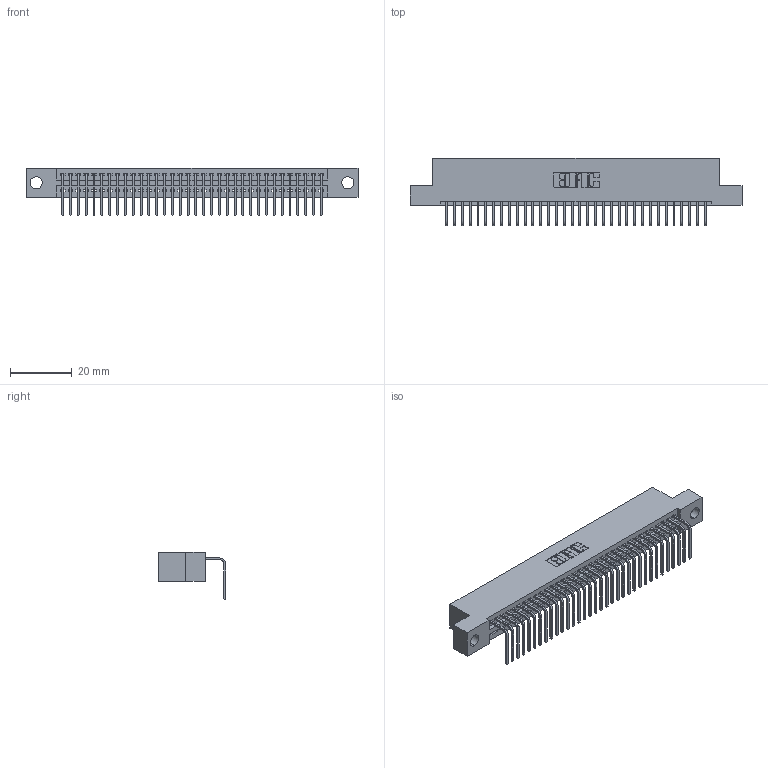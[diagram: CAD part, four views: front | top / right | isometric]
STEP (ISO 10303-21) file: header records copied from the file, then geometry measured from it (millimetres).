
FILE_DESCRIPTION (( 'STEP AP203' ), '1' );
FILE_NAME ('345-034-558-104.STEP', '2021-06-09T16:31:22', ( '' ), ( '' ), 'SwSTEP 2.0', 'SolidWorks 2020', '' );
FILE_SCHEMA (( 'CONFIG_CONTROL_DESIGN' ));
Length unit declared in the file: inch
Products named in the file (3): 345-034-558-104; 345 Part_Flush Mounting Lugs - 0.156 Dia-TI; 345-292-001_558 Tail - 2
Assembly tree (35 placements, depth 2):
  345-034-558-104
    345 Part_Flush Mounting Lugs - 0.156 Dia-TI
    345-292-001_558 Tail - 2  x34
Bounding box: 107.57 x 21.83 x 15.37 mm (x, y, z)
Volume: 10158.8 mm3; surface area: 13899.5 mm2
Topology: 35 solids, 35 shells, 2180 faces, 6565 edges, 4330 vertices
Faces by surface type: plane 1522, cylinder 658
Entity records: 27169 total; most frequent: CARTESIAN_POINT 4716, ORIENTED_EDGE 4682, DIRECTION 4129, EDGE_CURVE 2341, LINE 2073, VECTOR 2073, VERTEX_POINT 1558, AXIS2_PLACEMENT_3D 1028
